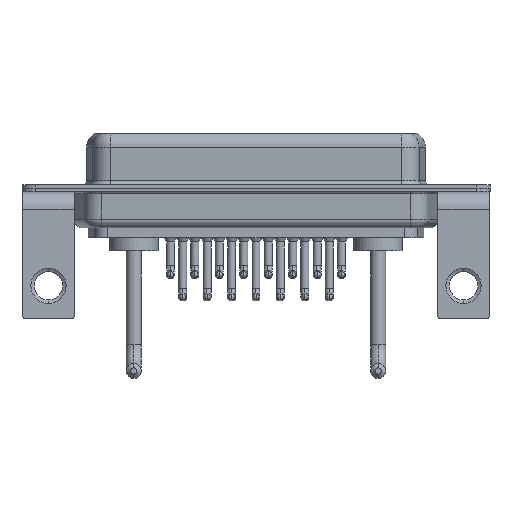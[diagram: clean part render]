
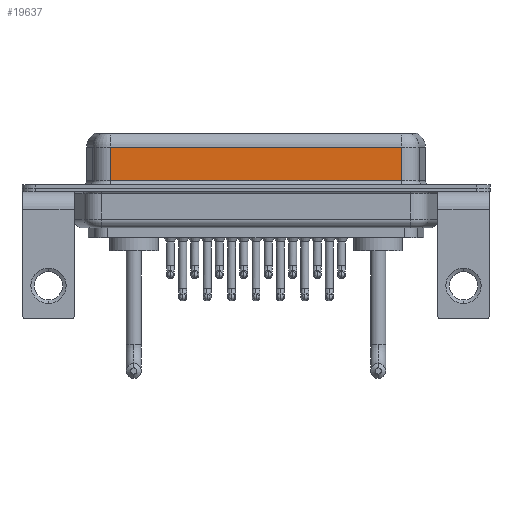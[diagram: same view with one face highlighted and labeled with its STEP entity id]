
A CAD part, front view. The second image highlights one B-rep face of the part: STEP entity #19637.
In plain terms, the highlighted planar face has unit normal (0, -1, 0).
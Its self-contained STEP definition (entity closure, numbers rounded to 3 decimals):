
#391 = AXIS2_PLACEMENT_3D ( 'NONE', #13082, #3224, #21482 ) ;
#573 = CARTESIAN_POINT ( 'NONE',  ( 7.013, -3.95, 0.9 ) ) ;
#1013 = VECTOR ( 'NONE', #18784, 1000. ) ;
#1664 = LINE ( 'NONE', #15236, #9120 ) ;
#2794 = LINE ( 'NONE', #8175, #20693 ) ;
#2987 = CARTESIAN_POINT ( 'NONE',  ( 40.037, -3.95, 0.9 ) ) ;
#3004 = FACE_OUTER_BOUND ( 'NONE', #13456, .T. ) ;
#3224 = DIRECTION ( 'NONE',  ( 0., 1., 0. ) ) ;
#4282 = ORIENTED_EDGE ( 'NONE', *, *, #17770, .T. ) ;
#4708 = ORIENTED_EDGE ( 'NONE', *, *, #8443, .T. ) ;
#4757 = VERTEX_POINT ( 'NONE', #573 ) ;
#5143 = CARTESIAN_POINT ( 'NONE',  ( 40.037, -3.95, 0.9 ) ) ;
#8033 = DIRECTION ( 'NONE',  ( 1., 0., 0. ) ) ;
#8175 = CARTESIAN_POINT ( 'NONE',  ( 7.013, -3.95, 6.4 ) ) ;
#8443 = EDGE_CURVE ( 'NONE', #21444, #4757, #2794, .T. ) ;
#8943 = LINE ( 'NONE', #12121, #1013 ) ;
#9043 = ORIENTED_EDGE ( 'NONE', *, *, #10215, .T. ) ;
#9120 = VECTOR ( 'NONE', #18193, 1000. ) ;
#9490 = DIRECTION ( 'NONE',  ( 0., 0., -1. ) ) ;
#10215 = EDGE_CURVE ( 'NONE', #4757, #15055, #21142, .T. ) ;
#10629 = CARTESIAN_POINT ( 'NONE',  ( 40.037, -3.95, 4.65 ) ) ;
#10811 = VERTEX_POINT ( 'NONE', #10629 ) ;
#12121 = CARTESIAN_POINT ( 'NONE',  ( 40.037, -3.95, 6.4 ) ) ;
#12447 = EDGE_CURVE ( 'NONE', #10811, #15055, #8943, .T. ) ;
#13082 = CARTESIAN_POINT ( 'NONE',  ( 40.037, -3.95, 6.4 ) ) ;
#13280 = VECTOR ( 'NONE', #8033, 1000. ) ;
#13300 = PLANE ( 'NONE',  #391 ) ;
#13456 = EDGE_LOOP ( 'NONE', ( #17103, #4282, #4708, #9043 ) ) ;
#15055 = VERTEX_POINT ( 'NONE', #5143 ) ;
#15236 = CARTESIAN_POINT ( 'NONE',  ( 40.037, -3.95, 4.65 ) ) ;
#17103 = ORIENTED_EDGE ( 'NONE', *, *, #12447, .F. ) ;
#17770 = EDGE_CURVE ( 'NONE', #10811, #21444, #1664, .T. ) ;
#18193 = DIRECTION ( 'NONE',  ( -1., 0., 0. ) ) ;
#18784 = DIRECTION ( 'NONE',  ( 0., 0., -1. ) ) ;
#19637 = ADVANCED_FACE ( 'NONE', ( #3004 ), #13300, .F. ) ;
#20248 = CARTESIAN_POINT ( 'NONE',  ( 7.013, -3.95, 4.65 ) ) ;
#20693 = VECTOR ( 'NONE', #9490, 1000. ) ;
#21142 = LINE ( 'NONE', #2987, #13280 ) ;
#21444 = VERTEX_POINT ( 'NONE', #20248 ) ;
#21482 = DIRECTION ( 'NONE',  ( 0., 0., 1. ) ) ;
